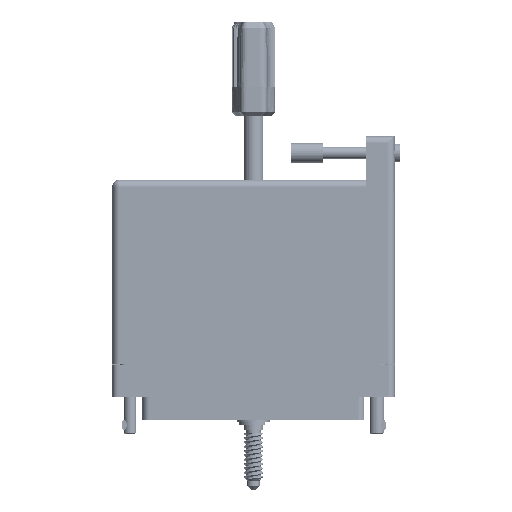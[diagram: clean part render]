
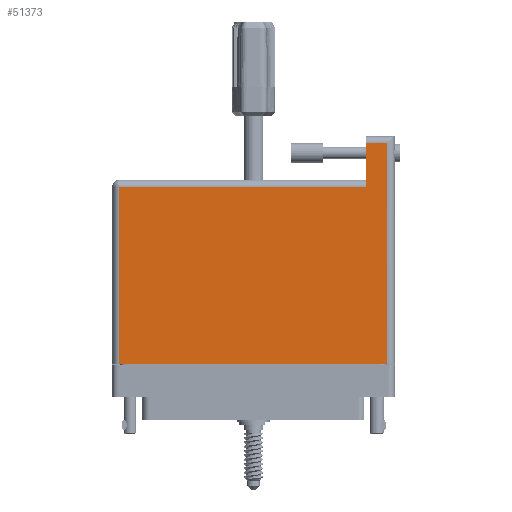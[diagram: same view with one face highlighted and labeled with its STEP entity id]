
A CAD part, front view. The second image highlights one B-rep face of the part: STEP entity #51373.
In plain terms, the highlighted face is planar.
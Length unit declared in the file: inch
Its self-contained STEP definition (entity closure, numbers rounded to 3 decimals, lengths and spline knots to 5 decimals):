
#1075 = CARTESIAN_POINT ( 'NONE',  ( 1.289, 2.095, 0.617 ) ) ;
#2604 = LINE ( 'NONE', #19515, #20173 ) ;
#5026 = LINE ( 'NONE', #19810, #82136 ) ;
#5836 = CARTESIAN_POINT ( 'NONE',  ( -1.359, 2.025, 0.617 ) ) ;
#9592 = VERTEX_POINT ( 'NONE', #34544 ) ;
#15339 = CARTESIAN_POINT ( 'NONE',  ( -1.359, -0.1, 0.617 ) ) ;
#15793 = CARTESIAN_POINT ( 'NONE',  ( -1.289, 1.605, 0.617 ) ) ;
#18273 = VECTOR ( 'NONE', #46500, 39.37008 ) ;
#19515 = CARTESIAN_POINT ( 'NONE',  ( -1.359, 1.605, 0.617 ) ) ;
#19810 = CARTESIAN_POINT ( 'NONE',  ( 1.079, 2.095, 0.617 ) ) ;
#20140 = DIRECTION ( 'NONE',  ( 0., -1., 0. ) ) ;
#20173 = VECTOR ( 'NONE', #50192, 39.37008 ) ;
#22811 = ORIENTED_EDGE ( 'NONE', *, *, #41840, .T. ) ;
#24156 = EDGE_CURVE ( 'NONE', #94535, #44552, #25366, .T. ) ;
#25366 = LINE ( 'NONE', #1075, #18273 ) ;
#29948 = CARTESIAN_POINT ( 'NONE',  ( -1.359, 1.675, 0.617 ) ) ;
#29959 = CARTESIAN_POINT ( 'NONE',  ( 1.289, -0.1, 0.617 ) ) ;
#29974 = ORIENTED_EDGE ( 'NONE', *, *, #95705, .T. ) ;
#30497 = VERTEX_POINT ( 'NONE', #15793 ) ;
#32989 = CARTESIAN_POINT ( 'NONE',  ( -1.289, -0.1, 0.617 ) ) ;
#34424 = LINE ( 'NONE', #5836, #79904 ) ;
#34544 = CARTESIAN_POINT ( 'NONE',  ( 1.079, 1.605, 0.617 ) ) ;
#36427 = VECTOR ( 'NONE', #45042, 39.37008 ) ;
#41840 = EDGE_CURVE ( 'NONE', #30497, #68288, #85657, .T. ) ;
#42830 = EDGE_CURVE ( 'NONE', #68288, #94535, #60933, .T. ) ;
#43204 = FACE_OUTER_BOUND ( 'NONE', #75653, .T. ) ;
#44552 = VERTEX_POINT ( 'NONE', #52392 ) ;
#45042 = DIRECTION ( 'NONE',  ( 1., 0., 0. ) ) ;
#46500 = DIRECTION ( 'NONE',  ( 0., 1., 0. ) ) ;
#47394 = CARTESIAN_POINT ( 'NONE',  ( 1.079, 2.025, 0.617 ) ) ;
#47831 = ORIENTED_EDGE ( 'NONE', *, *, #83341, .T. ) ;
#48320 = ORIENTED_EDGE ( 'NONE', *, *, #24156, .T. ) ;
#50192 = DIRECTION ( 'NONE',  ( -1., 0., 0. ) ) ;
#51373 = ADVANCED_FACE ( 'NONE', ( #43204 ), #52751, .F. ) ;
#52392 = CARTESIAN_POINT ( 'NONE',  ( 1.289, 2.025, 0.617 ) ) ;
#52530 = ORIENTED_EDGE ( 'NONE', *, *, #42830, .T. ) ;
#52751 = PLANE ( 'NONE',  #65301 ) ;
#57802 = DIRECTION ( 'NONE',  ( -1., 0., 0. ) ) ;
#59921 = DIRECTION ( 'NONE',  ( 0., 0., -1. ) ) ;
#60933 = LINE ( 'NONE', #15339, #36427 ) ;
#62558 = VERTEX_POINT ( 'NONE', #47394 ) ;
#65301 = AXIS2_PLACEMENT_3D ( 'NONE', #29948, #59921, #75573 ) ;
#65791 = VECTOR ( 'NONE', #93313, 39.37008 ) ;
#68288 = VERTEX_POINT ( 'NONE', #70081 ) ;
#70081 = CARTESIAN_POINT ( 'NONE',  ( -1.289, -0.1, 0.617 ) ) ;
#72537 = ORIENTED_EDGE ( 'NONE', *, *, #84750, .T. ) ;
#75573 = DIRECTION ( 'NONE',  ( -1., 0., 0. ) ) ;
#75653 = EDGE_LOOP ( 'NONE', ( #72537, #22811, #52530, #48320, #29974, #47831 ) ) ;
#79904 = VECTOR ( 'NONE', #57802, 39.37008 ) ;
#82136 = VECTOR ( 'NONE', #20140, 39.37008 ) ;
#83341 = EDGE_CURVE ( 'NONE', #62558, #9592, #5026, .T. ) ;
#84750 = EDGE_CURVE ( 'NONE', #9592, #30497, #2604, .T. ) ;
#85657 = LINE ( 'NONE', #32989, #65791 ) ;
#93313 = DIRECTION ( 'NONE',  ( 0., -1., 0. ) ) ;
#94535 = VERTEX_POINT ( 'NONE', #29959 ) ;
#95705 = EDGE_CURVE ( 'NONE', #44552, #62558, #34424, .T. ) ;
